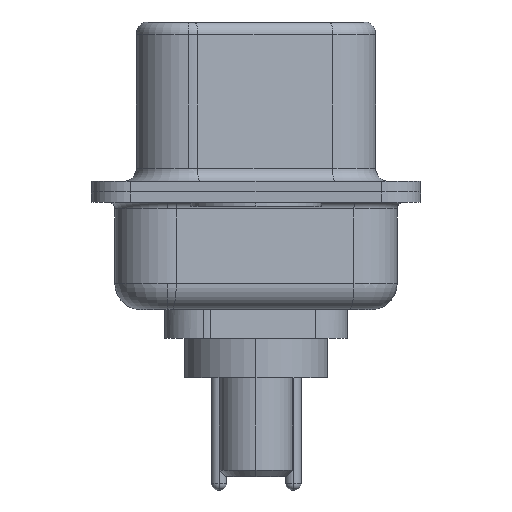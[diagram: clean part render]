
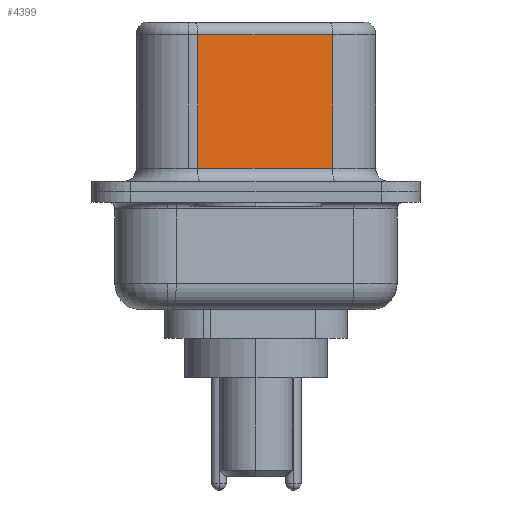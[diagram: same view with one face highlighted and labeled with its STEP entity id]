
A CAD part, left-side view. The second image highlights one B-rep face of the part: STEP entity #4399.
In plain terms, the highlighted planar face has unit normal (-0.985, -0.174, 0).
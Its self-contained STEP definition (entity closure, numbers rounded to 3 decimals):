
#255 = CARTESIAN_POINT ( 'NONE',  ( 4.585, -2.927, 6.52 ) ) ;
#526 = ORIENTED_EDGE ( 'NONE', *, *, #12308, .T. ) ;
#2281 = CARTESIAN_POINT ( 'NONE',  ( 3.675, 2.233, 6.52 ) ) ;
#2705 = VECTOR ( 'NONE', #7626, 1000. ) ;
#2739 = VECTOR ( 'NONE', #5262, 1000. ) ;
#4399 = ADVANCED_FACE ( 'NONE', ( #14170 ), #15093, .F. ) ;
#4502 = VECTOR ( 'NONE', #11041, 1000. ) ;
#4993 = CARTESIAN_POINT ( 'NONE',  ( 4.585, -2.927, 6.52 ) ) ;
#5191 = VERTEX_POINT ( 'NONE', #10511 ) ;
#5262 = DIRECTION ( 'NONE',  ( -0.174, 0.985, 0. ) ) ;
#5516 = LINE ( 'NONE', #13573, #2705 ) ;
#5802 = VERTEX_POINT ( 'NONE', #9023 ) ;
#5969 = ORIENTED_EDGE ( 'NONE', *, *, #13294, .T. ) ;
#6857 = AXIS2_PLACEMENT_3D ( 'NONE', #255, #10766, #6867 ) ;
#6867 = DIRECTION ( 'NONE',  ( -0.174, 0.985, 0. ) ) ;
#7509 = EDGE_CURVE ( 'NONE', #14407, #5802, #13900, .T. ) ;
#7626 = DIRECTION ( 'NONE',  ( 0.174, -0.985, 0. ) ) ;
#8218 = VERTEX_POINT ( 'NONE', #9509 ) ;
#8264 = VECTOR ( 'NONE', #11724, 1000. ) ;
#8925 = CARTESIAN_POINT ( 'NONE',  ( 4.585, -2.927, 6.02 ) ) ;
#9023 = CARTESIAN_POINT ( 'NONE',  ( 4.585, -2.927, 0.9 ) ) ;
#9509 = CARTESIAN_POINT ( 'NONE',  ( 3.675, 2.233, 0.9 ) ) ;
#10511 = CARTESIAN_POINT ( 'NONE',  ( 3.675, 2.233, 6.02 ) ) ;
#10747 = EDGE_CURVE ( 'NONE', #5191, #8218, #14555, .T. ) ;
#10766 = DIRECTION ( 'NONE',  ( 0.985, 0.174, 0. ) ) ;
#11041 = DIRECTION ( 'NONE',  ( 0., 0., -1. ) ) ;
#11104 = CARTESIAN_POINT ( 'NONE',  ( 4.585, -2.927, 6.02 ) ) ;
#11724 = DIRECTION ( 'NONE',  ( 0., 0., -1. ) ) ;
#12308 = EDGE_CURVE ( 'NONE', #14407, #5191, #15304, .T. ) ;
#13294 = EDGE_CURVE ( 'NONE', #8218, #5802, #5516, .T. ) ;
#13573 = CARTESIAN_POINT ( 'NONE',  ( 4.585, -2.927, 0.9 ) ) ;
#13687 = ORIENTED_EDGE ( 'NONE', *, *, #10747, .T. ) ;
#13900 = LINE ( 'NONE', #4993, #4502 ) ;
#14170 = FACE_OUTER_BOUND ( 'NONE', #15068, .T. ) ;
#14407 = VERTEX_POINT ( 'NONE', #8925 ) ;
#14431 = ORIENTED_EDGE ( 'NONE', *, *, #7509, .F. ) ;
#14555 = LINE ( 'NONE', #2281, #8264 ) ;
#15068 = EDGE_LOOP ( 'NONE', ( #14431, #526, #13687, #5969 ) ) ;
#15093 = PLANE ( 'NONE',  #6857 ) ;
#15304 = LINE ( 'NONE', #11104, #2739 ) ;
